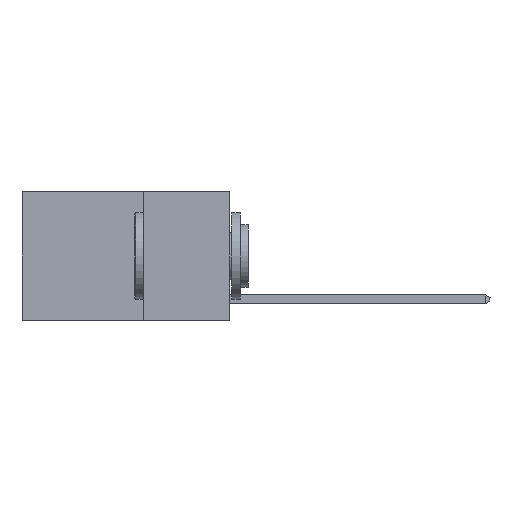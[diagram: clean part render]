
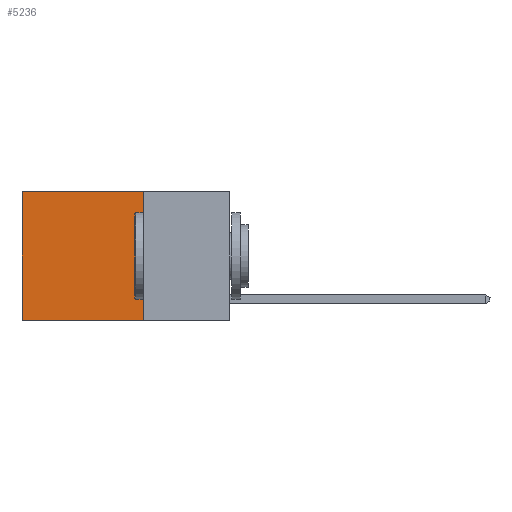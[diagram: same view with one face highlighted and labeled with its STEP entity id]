
A CAD part, left-side view. The second image highlights one B-rep face of the part: STEP entity #5236.
In plain terms, the highlighted planar face has unit normal (-1, 0, 0).
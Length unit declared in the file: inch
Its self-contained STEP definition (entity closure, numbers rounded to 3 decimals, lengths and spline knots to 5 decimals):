
#2445 = DIRECTION ( 'NONE',  ( 0., 0., -1. ) ) ;
#2756 = VERTEX_POINT ( 'NONE', #13249 ) ;
#3091 = LINE ( 'NONE', #16836, #22254 ) ;
#3383 = LINE ( 'NONE', #18919, #23986 ) ;
#3418 = ORIENTED_EDGE ( 'NONE', *, *, #3906, .T. ) ;
#3906 = EDGE_CURVE ( 'NONE', #17250, #11204, #3091, .T. ) ;
#4425 = AXIS2_PLACEMENT_3D ( 'NONE', #8747, #5049, #12921 ) ;
#4499 = ORIENTED_EDGE ( 'NONE', *, *, #10306, .F. ) ;
#5049 = DIRECTION ( 'NONE',  ( 1., 0., 0. ) ) ;
#5236 = ADVANCED_FACE ( 'NONE', ( #18166 ), #8622, .F. ) ;
#6078 = EDGE_LOOP ( 'NONE', ( #18534, #4499, #7939, #3418 ) ) ;
#6939 = DIRECTION ( 'NONE',  ( 0., 0., -1. ) ) ;
#7061 = DIRECTION ( 'NONE',  ( 0., 1., 0. ) ) ;
#7939 = ORIENTED_EDGE ( 'NONE', *, *, #24948, .F. ) ;
#8622 = PLANE ( 'NONE',  #4425 ) ;
#8747 = CARTESIAN_POINT ( 'NONE',  ( 0.2625, 0.25, 0. ) ) ;
#8876 = DIRECTION ( 'NONE',  ( 0., 1., 0. ) ) ;
#8921 = VERTEX_POINT ( 'NONE', #15988 ) ;
#10306 = EDGE_CURVE ( 'NONE', #2756, #8921, #3383, .T. ) ;
#11204 = VERTEX_POINT ( 'NONE', #13512 ) ;
#12384 = LINE ( 'NONE', #20180, #15534 ) ;
#12921 = DIRECTION ( 'NONE',  ( 0., 0., -1. ) ) ;
#13249 = CARTESIAN_POINT ( 'NONE',  ( 0.2625, 0.25, -0.37 ) ) ;
#13512 = CARTESIAN_POINT ( 'NONE',  ( 0.2625, 0.6, 0. ) ) ;
#13972 = VECTOR ( 'NONE', #6939, 39.37008 ) ;
#14946 = CARTESIAN_POINT ( 'NONE',  ( 0.2625, 0.25, 0. ) ) ;
#15534 = VECTOR ( 'NONE', #2445, 39.37008 ) ;
#15988 = CARTESIAN_POINT ( 'NONE',  ( 0.2625, 0.6, -0.37 ) ) ;
#16836 = CARTESIAN_POINT ( 'NONE',  ( 0.2625, 0.25, 0. ) ) ;
#17250 = VERTEX_POINT ( 'NONE', #14946 ) ;
#18166 = FACE_OUTER_BOUND ( 'NONE', #6078, .T. ) ;
#18389 = CARTESIAN_POINT ( 'NONE',  ( 0.2625, 0.25, 0. ) ) ;
#18534 = ORIENTED_EDGE ( 'NONE', *, *, #21577, .T. ) ;
#18919 = CARTESIAN_POINT ( 'NONE',  ( 0.2625, 0.25, -0.37 ) ) ;
#20180 = CARTESIAN_POINT ( 'NONE',  ( 0.2625, 0.6, 0. ) ) ;
#20810 = LINE ( 'NONE', #18389, #13972 ) ;
#21577 = EDGE_CURVE ( 'NONE', #11204, #8921, #12384, .T. ) ;
#22254 = VECTOR ( 'NONE', #7061, 39.37008 ) ;
#23986 = VECTOR ( 'NONE', #8876, 39.37008 ) ;
#24948 = EDGE_CURVE ( 'NONE', #17250, #2756, #20810, .T. ) ;
